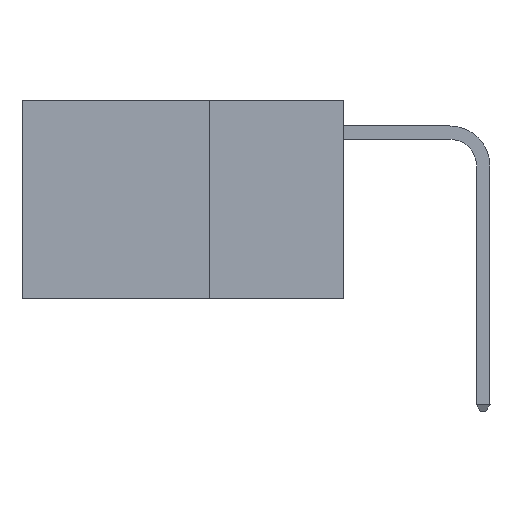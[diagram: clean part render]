
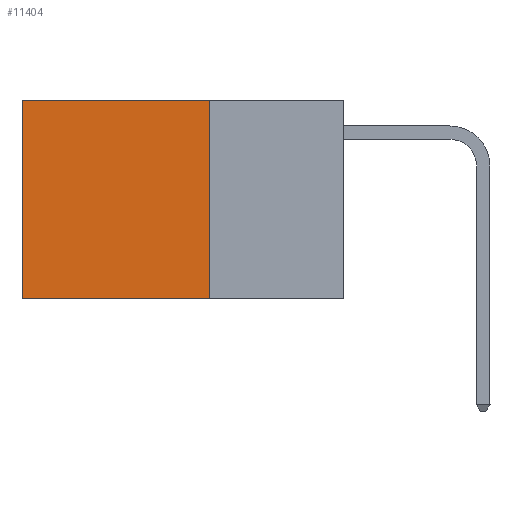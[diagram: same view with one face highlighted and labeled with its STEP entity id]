
A CAD part, left-side view. The second image highlights one B-rep face of the part: STEP entity #11404.
In plain terms, the highlighted planar face has unit normal (-1, 0, 0).
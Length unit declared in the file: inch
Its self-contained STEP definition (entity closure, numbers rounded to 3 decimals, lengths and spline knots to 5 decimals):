
#237 = CARTESIAN_POINT ( 'NONE',  ( 0.2625, 0.25, 0. ) ) ;
#1419 = CARTESIAN_POINT ( 'NONE',  ( 0.2625, 0.6, -0.37 ) ) ;
#2433 = VECTOR ( 'NONE', #10933, 39.37008 ) ;
#2512 = LINE ( 'NONE', #7763, #15299 ) ;
#2550 = CARTESIAN_POINT ( 'NONE',  ( 0.2625, 0.25, 0. ) ) ;
#3583 = VECTOR ( 'NONE', #11443, 39.37008 ) ;
#3811 = VERTEX_POINT ( 'NONE', #11035 ) ;
#3947 = ORIENTED_EDGE ( 'NONE', *, *, #8240, .F. ) ;
#4082 = CARTESIAN_POINT ( 'NONE',  ( 0.2625, 0.25, 0. ) ) ;
#4945 = LINE ( 'NONE', #5007, #14429 ) ;
#5007 = CARTESIAN_POINT ( 'NONE',  ( 0.2625, 0.25, -0.37 ) ) ;
#5361 = DIRECTION ( 'NONE',  ( 1., 0., 0. ) ) ;
#5686 = EDGE_CURVE ( 'NONE', #3811, #8869, #12361, .T. ) ;
#6374 = VERTEX_POINT ( 'NONE', #2550 ) ;
#6373 = EDGE_LOOP ( 'NONE', ( #8954, #15633, #3947, #6875 ) ) ;
#6488 = LINE ( 'NONE', #237, #3583 ) ;
#6875 = ORIENTED_EDGE ( 'NONE', *, *, #10753, .T. ) ;
#7763 = CARTESIAN_POINT ( 'NONE',  ( 0.2625, 0.25, 0. ) ) ;
#8240 = EDGE_CURVE ( 'NONE', #6374, #10472, #2512, .T. ) ;
#8388 = AXIS2_PLACEMENT_3D ( 'NONE', #4082, #5361, #14007 ) ;
#8869 = VERTEX_POINT ( 'NONE', #1419 ) ;
#8943 = PLANE ( 'NONE',  #8388 ) ;
#8954 = ORIENTED_EDGE ( 'NONE', *, *, #5686, .T. ) ;
#9005 = DIRECTION ( 'NONE',  ( 0., 0., -1. ) ) ;
#9636 = CARTESIAN_POINT ( 'NONE',  ( 0.2625, 0.25, -0.37 ) ) ;
#10472 = VERTEX_POINT ( 'NONE', #9636 ) ;
#10753 = EDGE_CURVE ( 'NONE', #6374, #3811, #6488, .T. ) ;
#10933 = DIRECTION ( 'NONE',  ( 0., 0., -1. ) ) ;
#10944 = CARTESIAN_POINT ( 'NONE',  ( 0.2625, 0.6, 0. ) ) ;
#11035 = CARTESIAN_POINT ( 'NONE',  ( 0.2625, 0.6, 0. ) ) ;
#11404 = ADVANCED_FACE ( 'NONE', ( #13479 ), #8943, .F. ) ;
#11443 = DIRECTION ( 'NONE',  ( 0., 1., 0. ) ) ;
#11554 = EDGE_CURVE ( 'NONE', #10472, #8869, #4945, .T. ) ;
#12361 = LINE ( 'NONE', #10944, #2433 ) ;
#13479 = FACE_OUTER_BOUND ( 'NONE', #6373, .T. ) ;
#14007 = DIRECTION ( 'NONE',  ( 0., 0., -1. ) ) ;
#14429 = VECTOR ( 'NONE', #16139, 39.37008 ) ;
#15299 = VECTOR ( 'NONE', #9005, 39.37008 ) ;
#15633 = ORIENTED_EDGE ( 'NONE', *, *, #11554, .F. ) ;
#16139 = DIRECTION ( 'NONE',  ( 0., 1., 0. ) ) ;
